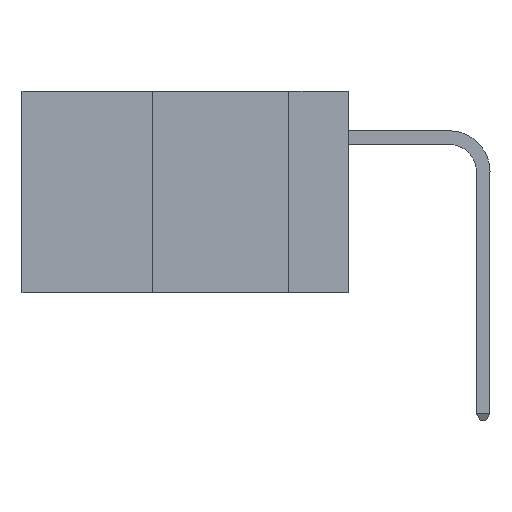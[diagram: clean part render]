
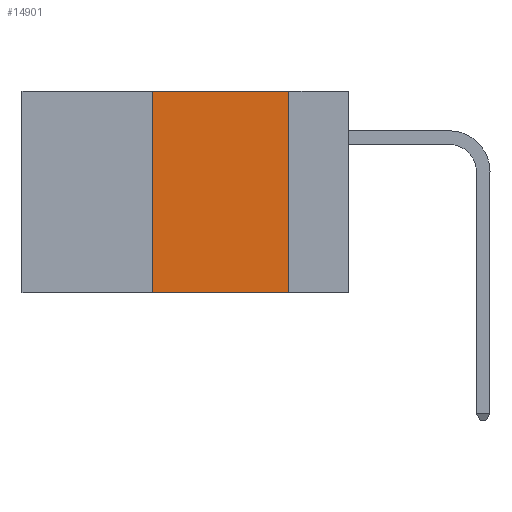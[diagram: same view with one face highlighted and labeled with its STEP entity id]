
A CAD part, left-side view. The second image highlights one B-rep face of the part: STEP entity #14901.
In plain terms, the highlighted planar face has unit normal (-1, 0, 0).
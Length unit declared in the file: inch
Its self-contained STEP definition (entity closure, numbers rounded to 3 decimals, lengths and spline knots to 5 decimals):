
#275 = VERTEX_POINT ( 'NONE', #1894 ) ;
#1609 = ORIENTED_EDGE ( 'NONE', *, *, #4939, .F. ) ;
#1894 = CARTESIAN_POINT ( 'NONE',  ( 0., 0.11, 0. ) ) ;
#2205 = DIRECTION ( 'NONE',  ( 0., 0., -1. ) ) ;
#2720 = VERTEX_POINT ( 'NONE', #28365 ) ;
#2820 = DIRECTION ( 'NONE',  ( 0., 0., 1. ) ) ;
#3170 = CARTESIAN_POINT ( 'NONE',  ( 0., 0.6, 0. ) ) ;
#3417 = AXIS2_PLACEMENT_3D ( 'NONE', #3170, #20290, #5637 ) ;
#4269 = EDGE_CURVE ( 'NONE', #275, #2720, #12513, .T. ) ;
#4823 = CARTESIAN_POINT ( 'NONE',  ( 0., 0.36, 0. ) ) ;
#4939 = EDGE_CURVE ( 'NONE', #23769, #31460, #12090, .T. ) ;
#5448 = CARTESIAN_POINT ( 'NONE',  ( 0., 0.36, -0.37 ) ) ;
#5637 = DIRECTION ( 'NONE',  ( 0., 0., -1. ) ) ;
#6995 = ORIENTED_EDGE ( 'NONE', *, *, #13112, .F. ) ;
#8552 = ORIENTED_EDGE ( 'NONE', *, *, #22009, .T. ) ;
#10133 = CARTESIAN_POINT ( 'NONE',  ( 0., 0.11, 0. ) ) ;
#10370 = ORIENTED_EDGE ( 'NONE', *, *, #4269, .F. ) ;
#11276 = LINE ( 'NONE', #30667, #30806 ) ;
#12090 = LINE ( 'NONE', #12567, #17840 ) ;
#12513 = LINE ( 'NONE', #10133, #24786 ) ;
#12567 = CARTESIAN_POINT ( 'NONE',  ( 0., 0.36, 0. ) ) ;
#13112 = EDGE_CURVE ( 'NONE', #31460, #275, #11276, .T. ) ;
#14676 = CARTESIAN_POINT ( 'NONE',  ( 0., 0.6, -0.37 ) ) ;
#14901 = ADVANCED_FACE ( 'NONE', ( #21891 ), #27595, .F. ) ;
#16019 = DIRECTION ( 'NONE',  ( 0., -1., 0. ) ) ;
#17078 = VECTOR ( 'NONE', #17134, 39.37008 ) ;
#17134 = DIRECTION ( 'NONE',  ( 0., -1., 0. ) ) ;
#17840 = VECTOR ( 'NONE', #2820, 39.37008 ) ;
#20290 = DIRECTION ( 'NONE',  ( 1., 0., 0. ) ) ;
#21891 = FACE_OUTER_BOUND ( 'NONE', #23238, .T. ) ;
#22009 = EDGE_CURVE ( 'NONE', #23769, #2720, #30115, .T. ) ;
#23238 = EDGE_LOOP ( 'NONE', ( #10370, #6995, #1609, #8552 ) ) ;
#23769 = VERTEX_POINT ( 'NONE', #5448 ) ;
#24786 = VECTOR ( 'NONE', #2205, 39.37008 ) ;
#27595 = PLANE ( 'NONE',  #3417 ) ;
#28365 = CARTESIAN_POINT ( 'NONE',  ( 0., 0.11, -0.37 ) ) ;
#30115 = LINE ( 'NONE', #14676, #17078 ) ;
#30667 = CARTESIAN_POINT ( 'NONE',  ( 0., 0.6, 0. ) ) ;
#30806 = VECTOR ( 'NONE', #16019, 39.37008 ) ;
#31460 = VERTEX_POINT ( 'NONE', #4823 ) ;
